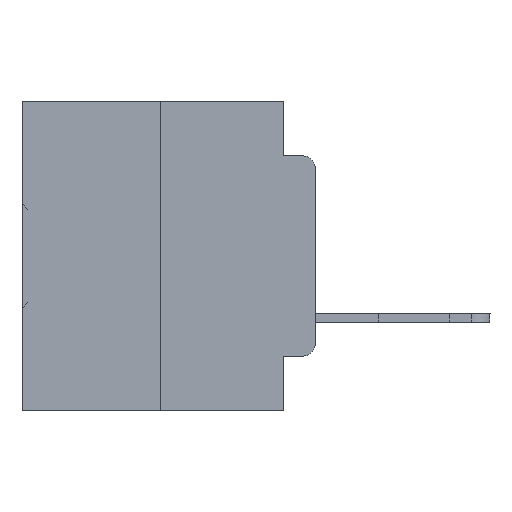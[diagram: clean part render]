
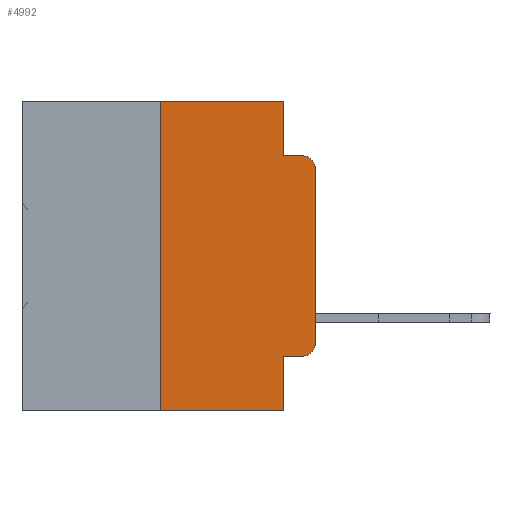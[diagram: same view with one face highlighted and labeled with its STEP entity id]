
A CAD part, left-side view. The second image highlights one B-rep face of the part: STEP entity #4992.
In plain terms, the highlighted planar face has unit normal (-1, 0, 0).
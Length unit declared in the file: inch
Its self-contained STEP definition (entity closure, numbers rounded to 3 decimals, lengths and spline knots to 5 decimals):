
#158 = EDGE_CURVE ( 'NONE', #5695, #33028, #30343, .T. ) ;
#198 = AXIS2_PLACEMENT_3D ( 'NONE', #22017, #5286, #19183 ) ;
#871 = EDGE_CURVE ( 'NONE', #22564, #33028, #31769, .T. ) ;
#876 = VERTEX_POINT ( 'NONE', #8827 ) ;
#923 = EDGE_CURVE ( 'NONE', #22564, #876, #25734, .T. ) ;
#975 = CARTESIAN_POINT ( 'NONE',  ( 0., 0.051, -0.4115 ) ) ;
#1460 = VECTOR ( 'NONE', #22554, 39.37008 ) ;
#1674 = DIRECTION ( 'NONE',  ( -1., 0., 0. ) ) ;
#2398 = EDGE_CURVE ( 'NONE', #29016, #11993, #22701, .T. ) ;
#2424 = ORIENTED_EDGE ( 'NONE', *, *, #7554, .T. ) ;
#2472 = AXIS2_PLACEMENT_3D ( 'NONE', #2825, #20090, #34776 ) ;
#2825 = CARTESIAN_POINT ( 'NONE',  ( 0., 0.473, 0. ) ) ;
#3110 = AXIS2_PLACEMENT_3D ( 'NONE', #21929, #1674, #15740 ) ;
#3184 = ORIENTED_EDGE ( 'NONE', *, *, #21834, .F. ) ;
#3796 = EDGE_CURVE ( 'NONE', #10877, #21778, #18693, .T. ) ;
#4374 = EDGE_CURVE ( 'NONE', #32104, #29016, #36380, .T. ) ;
#4588 = DIRECTION ( 'NONE',  ( 0., -1., 0. ) ) ;
#4992 = ADVANCED_FACE ( 'NONE', ( #8622 ), #13881, .F. ) ;
#5286 = DIRECTION ( 'NONE',  ( -1., 0., 0. ) ) ;
#5637 = DIRECTION ( 'NONE',  ( 0., 0., -1. ) ) ;
#5695 = VERTEX_POINT ( 'NONE', #24900 ) ;
#5865 = CARTESIAN_POINT ( 'NONE',  ( 0., 0.473, 0. ) ) ;
#6774 = ORIENTED_EDGE ( 'NONE', *, *, #3796, .T. ) ;
#6804 = CARTESIAN_POINT ( 'NONE',  ( 0., 0.051, 0. ) ) ;
#7554 = EDGE_CURVE ( 'NONE', #28107, #10877, #34163, .T. ) ;
#8505 = VECTOR ( 'NONE', #23249, 39.37008 ) ;
#8622 = FACE_OUTER_BOUND ( 'NONE', #29647, .T. ) ;
#8701 = CARTESIAN_POINT ( 'NONE',  ( 0., 0.051, -0.0885 ) ) ;
#8827 = CARTESIAN_POINT ( 'NONE',  ( 0., 0.02, -0.4115 ) ) ;
#10421 = DIRECTION ( 'NONE',  ( 0., 0., 1. ) ) ;
#10782 = DIRECTION ( 'NONE',  ( 0., -1., 0. ) ) ;
#10877 = VERTEX_POINT ( 'NONE', #28477 ) ;
#11077 = CARTESIAN_POINT ( 'NONE',  ( 0., 0.051, -0.0885 ) ) ;
#11504 = ORIENTED_EDGE ( 'NONE', *, *, #2398, .F. ) ;
#11569 = VECTOR ( 'NONE', #10421, 39.37008 ) ;
#11715 = ORIENTED_EDGE ( 'NONE', *, *, #923, .T. ) ;
#11993 = VERTEX_POINT ( 'NONE', #8701 ) ;
#13246 = CARTESIAN_POINT ( 'NONE',  ( 0., 0.25, 0. ) ) ;
#13613 = VECTOR ( 'NONE', #4588, 39.37008 ) ;
#13881 = PLANE ( 'NONE',  #2472 ) ;
#15428 = ORIENTED_EDGE ( 'NONE', *, *, #4374, .F. ) ;
#15740 = DIRECTION ( 'NONE',  ( 0., 0., -1. ) ) ;
#16597 = VECTOR ( 'NONE', #28746, 39.37008 ) ;
#16942 = ORIENTED_EDGE ( 'NONE', *, *, #24398, .F. ) ;
#17350 = ORIENTED_EDGE ( 'NONE', *, *, #35765, .T. ) ;
#18693 = CIRCLE ( 'NONE', #3110, 0.02 ) ;
#18694 = CARTESIAN_POINT ( 'NONE',  ( 0., 0.02, -0.0885 ) ) ;
#18770 = CARTESIAN_POINT ( 'NONE',  ( 0., 0.051, -0.5 ) ) ;
#19173 = VECTOR ( 'NONE', #10782, 39.37008 ) ;
#19183 = DIRECTION ( 'NONE',  ( 0., 0., -1. ) ) ;
#20090 = DIRECTION ( 'NONE',  ( 1., 0., 0. ) ) ;
#20104 = CARTESIAN_POINT ( 'NONE',  ( 0., 0.051, -0.4115 ) ) ;
#21778 = VERTEX_POINT ( 'NONE', #18694 ) ;
#21791 = ORIENTED_EDGE ( 'NONE', *, *, #158, .T. ) ;
#21834 = EDGE_CURVE ( 'NONE', #5695, #32104, #25258, .T. ) ;
#21929 = CARTESIAN_POINT ( 'NONE',  ( 0., 0.02, -0.1085 ) ) ;
#22017 = CARTESIAN_POINT ( 'NONE',  ( 0., 0.02, -0.3915 ) ) ;
#22554 = DIRECTION ( 'NONE',  ( 0., -1., 0. ) ) ;
#22564 = VERTEX_POINT ( 'NONE', #975 ) ;
#22701 = LINE ( 'NONE', #27787, #29757 ) ;
#23249 = DIRECTION ( 'NONE',  ( 0., 0., 1. ) ) ;
#24398 = EDGE_CURVE ( 'NONE', #11993, #21778, #30848, .T. ) ;
#24900 = CARTESIAN_POINT ( 'NONE',  ( 0., 0.25, -0.5 ) ) ;
#25258 = LINE ( 'NONE', #13246, #11569 ) ;
#25734 = LINE ( 'NONE', #20104, #16597 ) ;
#27787 = CARTESIAN_POINT ( 'NONE',  ( 0., 0.051, 0. ) ) ;
#27973 = DIRECTION ( 'NONE',  ( 0., 0., -1. ) ) ;
#28107 = VERTEX_POINT ( 'NONE', #32754 ) ;
#28477 = CARTESIAN_POINT ( 'NONE',  ( 0., 0., -0.1085 ) ) ;
#28746 = DIRECTION ( 'NONE',  ( 0., -1., 0. ) ) ;
#28937 = CARTESIAN_POINT ( 'NONE',  ( 0., 0.051, 0. ) ) ;
#29016 = VERTEX_POINT ( 'NONE', #6804 ) ;
#29624 = CIRCLE ( 'NONE', #198, 0.02 ) ;
#29647 = EDGE_LOOP ( 'NONE', ( #2424, #6774, #16942, #11504, #15428, #3184, #21791, #32211, #11715, #17350 ) ) ;
#29757 = VECTOR ( 'NONE', #27973, 39.37008 ) ;
#29854 = CARTESIAN_POINT ( 'NONE',  ( 0., 0.25, 0. ) ) ;
#30343 = LINE ( 'NONE', #32624, #13613 ) ;
#30848 = LINE ( 'NONE', #11077, #1460 ) ;
#31769 = LINE ( 'NONE', #28937, #34569 ) ;
#32104 = VERTEX_POINT ( 'NONE', #29854 ) ;
#32211 = ORIENTED_EDGE ( 'NONE', *, *, #871, .F. ) ;
#32624 = CARTESIAN_POINT ( 'NONE',  ( 0., 0.473, -0.5 ) ) ;
#32754 = CARTESIAN_POINT ( 'NONE',  ( 0., 0., -0.3915 ) ) ;
#33028 = VERTEX_POINT ( 'NONE', #18770 ) ;
#34163 = LINE ( 'NONE', #34727, #8505 ) ;
#34569 = VECTOR ( 'NONE', #5637, 39.37008 ) ;
#34727 = CARTESIAN_POINT ( 'NONE',  ( 0., 0., 0. ) ) ;
#34776 = DIRECTION ( 'NONE',  ( 0., 0., -1. ) ) ;
#35765 = EDGE_CURVE ( 'NONE', #876, #28107, #29624, .T. ) ;
#36380 = LINE ( 'NONE', #5865, #19173 ) ;
